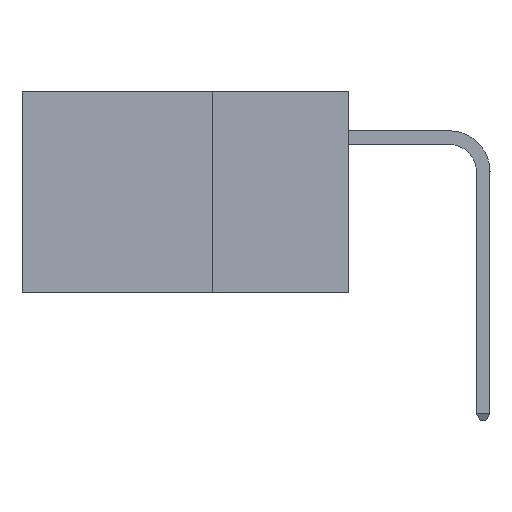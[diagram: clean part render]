
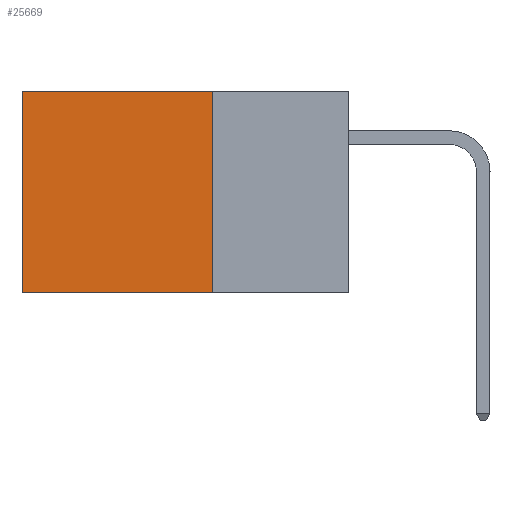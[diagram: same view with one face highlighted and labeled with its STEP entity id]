
A CAD part, left-side view. The second image highlights one B-rep face of the part: STEP entity #25669.
In plain terms, the highlighted planar face has unit normal (-1, 0, 0).
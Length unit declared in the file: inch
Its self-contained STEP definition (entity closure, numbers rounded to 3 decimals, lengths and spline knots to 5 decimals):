
#60 = VERTEX_POINT ( 'NONE', #17609 ) ;
#1285 = CARTESIAN_POINT ( 'NONE',  ( 0.2875, 0.25, 0. ) ) ;
#1397 = CARTESIAN_POINT ( 'NONE',  ( 0.2875, 0.25, 0. ) ) ;
#1603 = ORIENTED_EDGE ( 'NONE', *, *, #16698, .T. ) ;
#2015 = VERTEX_POINT ( 'NONE', #27032 ) ;
#2815 = EDGE_CURVE ( 'NONE', #16591, #60, #7854, .T. ) ;
#3345 = VECTOR ( 'NONE', #8724, 39.37008 ) ;
#4197 = DIRECTION ( 'NONE',  ( 0., 0., -1. ) ) ;
#5144 = VECTOR ( 'NONE', #16290, 39.37008 ) ;
#7854 = LINE ( 'NONE', #1285, #5144 ) ;
#8302 = LINE ( 'NONE', #23329, #3345 ) ;
#8393 = ORIENTED_EDGE ( 'NONE', *, *, #2815, .T. ) ;
#8724 = DIRECTION ( 'NONE',  ( 0., 0., -1. ) ) ;
#9489 = LINE ( 'NONE', #19851, #13524 ) ;
#10386 = FACE_OUTER_BOUND ( 'NONE', #20198, .T. ) ;
#11581 = LINE ( 'NONE', #1397, #15086 ) ;
#11651 = EDGE_CURVE ( 'NONE', #2015, #19173, #9489, .T. ) ;
#13524 = VECTOR ( 'NONE', #13653, 39.37008 ) ;
#13653 = DIRECTION ( 'NONE',  ( 0., 1., 0. ) ) ;
#14570 = CARTESIAN_POINT ( 'NONE',  ( 0.2875, 0.6, -0.37 ) ) ;
#15086 = VECTOR ( 'NONE', #16407, 39.37008 ) ;
#15976 = ORIENTED_EDGE ( 'NONE', *, *, #11651, .F. ) ;
#15977 = DIRECTION ( 'NONE',  ( 1., 0., 0. ) ) ;
#16290 = DIRECTION ( 'NONE',  ( 0., 1., 0. ) ) ;
#16407 = DIRECTION ( 'NONE',  ( 0., 0., -1. ) ) ;
#16591 = VERTEX_POINT ( 'NONE', #17013 ) ;
#16698 = EDGE_CURVE ( 'NONE', #60, #19173, #8302, .T. ) ;
#16757 = CARTESIAN_POINT ( 'NONE',  ( 0.2875, 0.25, 0. ) ) ;
#17013 = CARTESIAN_POINT ( 'NONE',  ( 0.2875, 0.25, 0. ) ) ;
#17609 = CARTESIAN_POINT ( 'NONE',  ( 0.2875, 0.6, 0. ) ) ;
#19173 = VERTEX_POINT ( 'NONE', #14570 ) ;
#19851 = CARTESIAN_POINT ( 'NONE',  ( 0.2875, 0.25, -0.37 ) ) ;
#20198 = EDGE_LOOP ( 'NONE', ( #1603, #15976, #22542, #8393 ) ) ;
#20244 = PLANE ( 'NONE',  #23860 ) ;
#22542 = ORIENTED_EDGE ( 'NONE', *, *, #25125, .F. ) ;
#23329 = CARTESIAN_POINT ( 'NONE',  ( 0.2875, 0.6, 0. ) ) ;
#23860 = AXIS2_PLACEMENT_3D ( 'NONE', #16757, #15977, #4197 ) ;
#25125 = EDGE_CURVE ( 'NONE', #16591, #2015, #11581, .T. ) ;
#25669 = ADVANCED_FACE ( 'NONE', ( #10386 ), #20244, .F. ) ;
#27032 = CARTESIAN_POINT ( 'NONE',  ( 0.2875, 0.25, -0.37 ) ) ;
